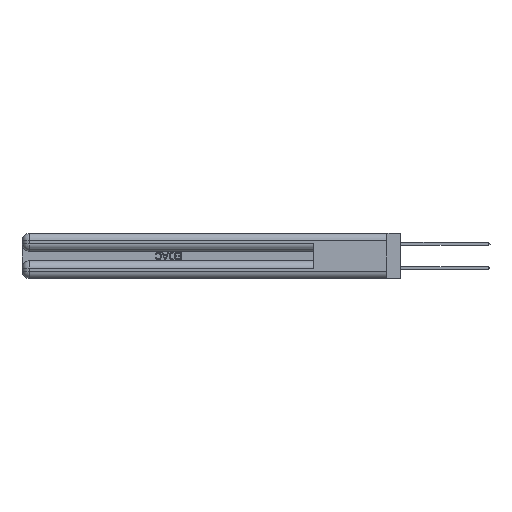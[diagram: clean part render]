
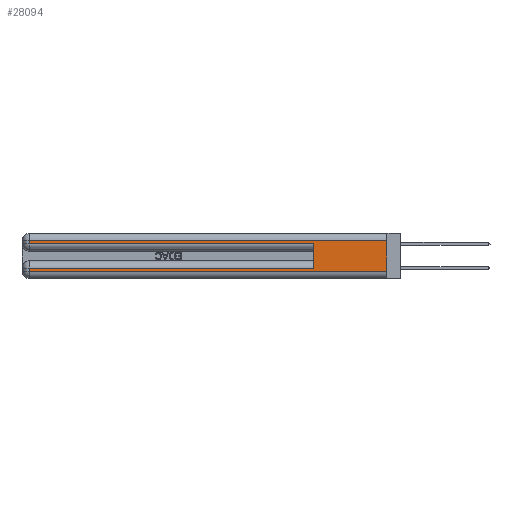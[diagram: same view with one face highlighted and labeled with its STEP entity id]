
A CAD part, left-side view. The second image highlights one B-rep face of the part: STEP entity #28094.
In plain terms, the highlighted planar face has unit normal (-1, 0, 0).
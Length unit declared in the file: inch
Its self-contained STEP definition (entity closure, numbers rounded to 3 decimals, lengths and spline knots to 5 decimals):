
#9 = LINE ( 'NONE', #31398, #29253 ) ;
#163 = EDGE_CURVE ( 'NONE', #40605, #22950, #20534, .T. ) ;
#4035 = VECTOR ( 'NONE', #27640, 39.37008 ) ;
#5438 = EDGE_CURVE ( 'NONE', #40748, #30558, #13762, .T. ) ;
#5648 = DIRECTION ( 'NONE',  ( 0., -1., 0. ) ) ;
#5751 = VECTOR ( 'NONE', #32867, 39.37008 ) ;
#6234 = EDGE_CURVE ( 'NONE', #8236, #8752, #27979, .T. ) ;
#8236 = VERTEX_POINT ( 'NONE', #11051 ) ;
#8752 = VERTEX_POINT ( 'NONE', #17423 ) ;
#9613 = VECTOR ( 'NONE', #5648, 39.37008 ) ;
#9744 = ORIENTED_EDGE ( 'NONE', *, *, #163, .T. ) ;
#9763 = ORIENTED_EDGE ( 'NONE', *, *, #5438, .T. ) ;
#11029 = CARTESIAN_POINT ( 'NONE',  ( 0., 0.6, 0.145 ) ) ;
#11051 = CARTESIAN_POINT ( 'NONE',  ( 0., 0., 0.31 ) ) ;
#11652 = CARTESIAN_POINT ( 'NONE',  ( 0., 0., 0.31 ) ) ;
#12129 = VECTOR ( 'NONE', #22635, 39.37008 ) ;
#12167 = CARTESIAN_POINT ( 'NONE',  ( 0., 0.6, 0.285 ) ) ;
#12335 = ORIENTED_EDGE ( 'NONE', *, *, #13213, .F. ) ;
#12404 = CARTESIAN_POINT ( 'NONE',  ( 0., 0., 0.37 ) ) ;
#13213 = EDGE_CURVE ( 'NONE', #23512, #22950, #15409, .T. ) ;
#13523 = CARTESIAN_POINT ( 'NONE',  ( 0., 2.94, 0.31 ) ) ;
#13762 = LINE ( 'NONE', #16640, #4035 ) ;
#15409 = LINE ( 'NONE', #11029, #5751 ) ;
#15897 = LINE ( 'NONE', #27486, #9613 ) ;
#16093 = DIRECTION ( 'NONE',  ( 1., 0., 0. ) ) ;
#16314 = CARTESIAN_POINT ( 'NONE',  ( 0., 2.94, 0.06 ) ) ;
#16640 = CARTESIAN_POINT ( 'NONE',  ( 0., 2.94, 0.37 ) ) ;
#17423 = CARTESIAN_POINT ( 'NONE',  ( 0., 0., 0.06 ) ) ;
#18133 = CARTESIAN_POINT ( 'NONE',  ( 0., 0., 0.37 ) ) ;
#18242 = VECTOR ( 'NONE', #36067, 39.37008 ) ;
#19899 = CARTESIAN_POINT ( 'NONE',  ( 0., 0., 0.285 ) ) ;
#20534 = LINE ( 'NONE', #19899, #29110 ) ;
#22635 = DIRECTION ( 'NONE',  ( 0., 1., 0. ) ) ;
#22950 = VERTEX_POINT ( 'NONE', #12167 ) ;
#23512 = VERTEX_POINT ( 'NONE', #34109 ) ;
#24675 = VECTOR ( 'NONE', #32253, 39.37008 ) ;
#25084 = CARTESIAN_POINT ( 'NONE',  ( 0., 2.94, 0.37 ) ) ;
#25120 = CARTESIAN_POINT ( 'NONE',  ( 0., 2.94, 0.085 ) ) ;
#26601 = ORIENTED_EDGE ( 'NONE', *, *, #30568, .T. ) ;
#27486 = CARTESIAN_POINT ( 'NONE',  ( 0., 0., 0.06 ) ) ;
#27640 = DIRECTION ( 'NONE',  ( 0., 0., -1. ) ) ;
#27979 = LINE ( 'NONE', #18133, #18242 ) ;
#28094 = ADVANCED_FACE ( 'NONE', ( #45775 ), #37853, .F. ) ;
#29110 = VECTOR ( 'NONE', #45297, 39.37008 ) ;
#29164 = EDGE_CURVE ( 'NONE', #8236, #44779, #43413, .T. ) ;
#29253 = VECTOR ( 'NONE', #45765, 39.37008 ) ;
#30558 = VERTEX_POINT ( 'NONE', #16314 ) ;
#30568 = EDGE_CURVE ( 'NONE', #30558, #8752, #15897, .T. ) ;
#31398 = CARTESIAN_POINT ( 'NONE',  ( 0., 0., 0.085 ) ) ;
#32253 = DIRECTION ( 'NONE',  ( 0., 0., -1. ) ) ;
#32867 = DIRECTION ( 'NONE',  ( 0., 0., 1. ) ) ;
#34109 = CARTESIAN_POINT ( 'NONE',  ( 0., 0.6, 0.085 ) ) ;
#34703 = EDGE_CURVE ( 'NONE', #44779, #40605, #46244, .T. ) ;
#35825 = ORIENTED_EDGE ( 'NONE', *, *, #6234, .F. ) ;
#35842 = EDGE_CURVE ( 'NONE', #23512, #40748, #9, .T. ) ;
#36067 = DIRECTION ( 'NONE',  ( 0., 0., -1. ) ) ;
#37853 = PLANE ( 'NONE',  #39553 ) ;
#39039 = ORIENTED_EDGE ( 'NONE', *, *, #29164, .T. ) ;
#39352 = ORIENTED_EDGE ( 'NONE', *, *, #34703, .T. ) ;
#39553 = AXIS2_PLACEMENT_3D ( 'NONE', #12404, #16093, #41506 ) ;
#39972 = CARTESIAN_POINT ( 'NONE',  ( 0., 2.94, 0.285 ) ) ;
#40605 = VERTEX_POINT ( 'NONE', #39972 ) ;
#40748 = VERTEX_POINT ( 'NONE', #25120 ) ;
#41415 = EDGE_LOOP ( 'NONE', ( #35825, #39039, #39352, #9744, #12335, #42407, #9763, #26601 ) ) ;
#41506 = DIRECTION ( 'NONE',  ( 0., 0., -1. ) ) ;
#42407 = ORIENTED_EDGE ( 'NONE', *, *, #35842, .T. ) ;
#43413 = LINE ( 'NONE', #11652, #12129 ) ;
#44779 = VERTEX_POINT ( 'NONE', #13523 ) ;
#45297 = DIRECTION ( 'NONE',  ( 0., -1., 0. ) ) ;
#45765 = DIRECTION ( 'NONE',  ( 0., 1., 0. ) ) ;
#45775 = FACE_OUTER_BOUND ( 'NONE', #41415, .T. ) ;
#46244 = LINE ( 'NONE', #25084, #24675 ) ;
